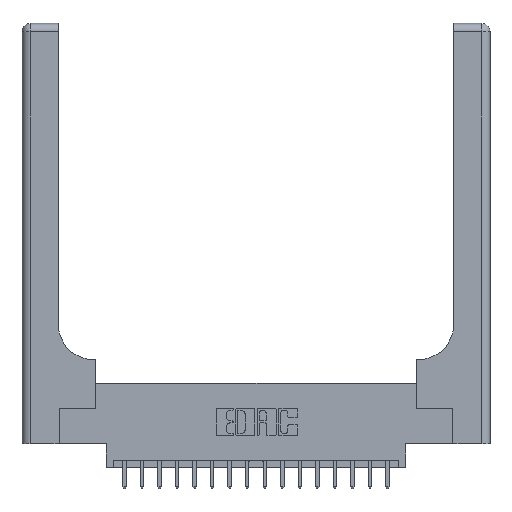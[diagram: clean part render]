
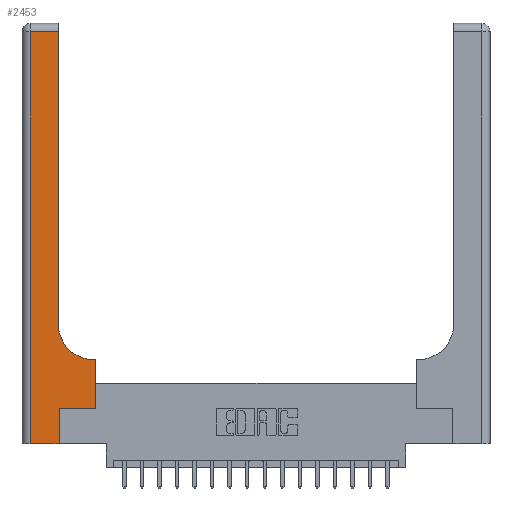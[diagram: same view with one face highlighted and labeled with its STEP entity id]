
A CAD part, top view. The second image highlights one B-rep face of the part: STEP entity #2453.
In plain terms, the highlighted planar face has unit normal (0, 0, 1).
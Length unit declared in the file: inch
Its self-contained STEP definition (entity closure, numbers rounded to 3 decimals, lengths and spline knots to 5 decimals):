
#224 = DIRECTION ( 'NONE',  ( 0., 1., 0. ) ) ;
#339 = CARTESIAN_POINT ( 'NONE',  ( 0.51, 0.85, 0.37 ) ) ;
#868 = VERTEX_POINT ( 'NONE', #2030 ) ;
#1755 = EDGE_CURVE ( 'NONE', #17602, #10268, #3141, .T. ) ;
#1922 = VECTOR ( 'NONE', #18468, 39.37008 ) ;
#1943 = CIRCLE ( 'NONE', #13120, 0.25 ) ;
#2030 = CARTESIAN_POINT ( 'NONE',  ( 0.528, 0.25, 0.37 ) ) ;
#2157 = CARTESIAN_POINT ( 'NONE',  ( 0.26, 2.94, 0.37 ) ) ;
#2203 = ORIENTED_EDGE ( 'NONE', *, *, #10490, .T. ) ;
#2453 = ADVANCED_FACE ( 'NONE', ( #17596 ), #16292, .F. ) ;
#2604 = CARTESIAN_POINT ( 'NONE',  ( 0., 3., 0.37 ) ) ;
#2752 = CARTESIAN_POINT ( 'NONE',  ( 0.265, 0.25, 0.37 ) ) ;
#2941 = VECTOR ( 'NONE', #11471, 39.37008 ) ;
#3141 = LINE ( 'NONE', #10660, #6651 ) ;
#3242 = ORIENTED_EDGE ( 'NONE', *, *, #4620, .T. ) ;
#4049 = CARTESIAN_POINT ( 'NONE',  ( 0., 0., 0.37 ) ) ;
#4089 = AXIS2_PLACEMENT_3D ( 'NONE', #2604, #8740, #15910 ) ;
#4101 = VERTEX_POINT ( 'NONE', #5188 ) ;
#4168 = VECTOR ( 'NONE', #9171, 39.37008 ) ;
#4620 = EDGE_CURVE ( 'NONE', #10268, #868, #8694, .T. ) ;
#4807 = VECTOR ( 'NONE', #8848, 39.37008 ) ;
#4898 = VERTEX_POINT ( 'NONE', #13884 ) ;
#5188 = CARTESIAN_POINT ( 'NONE',  ( 0.06, 2.94, 0.37 ) ) ;
#5408 = EDGE_LOOP ( 'NONE', ( #11699, #5452, #8083, #2203, #16127, #3242, #11478, #6878, #17930 ) ) ;
#5452 = ORIENTED_EDGE ( 'NONE', *, *, #7644, .T. ) ;
#5536 = CARTESIAN_POINT ( 'NONE',  ( 0.06, 3., 0.37 ) ) ;
#5556 = EDGE_CURVE ( 'NONE', #12656, #9653, #10816, .T. ) ;
#5921 = CARTESIAN_POINT ( 'NONE',  ( 0.06, 0., 0.37 ) ) ;
#6074 = VERTEX_POINT ( 'NONE', #2157 ) ;
#6420 = DIRECTION ( 'NONE',  ( 0., 0., -1. ) ) ;
#6651 = VECTOR ( 'NONE', #9278, 39.37008 ) ;
#6656 = EDGE_CURVE ( 'NONE', #4101, #14991, #19210, .T. ) ;
#6878 = ORIENTED_EDGE ( 'NONE', *, *, #5556, .T. ) ;
#7611 = LINE ( 'NONE', #18388, #17692 ) ;
#7644 = EDGE_CURVE ( 'NONE', #6074, #4101, #11165, .T. ) ;
#7708 = CARTESIAN_POINT ( 'NONE',  ( 0.26, 3., 0.37 ) ) ;
#8083 = ORIENTED_EDGE ( 'NONE', *, *, #6656, .T. ) ;
#8111 = CARTESIAN_POINT ( 'NONE',  ( 0.26, 0.6, 0.37 ) ) ;
#8381 = CARTESIAN_POINT ( 'NONE',  ( 0.528, 0.6, 0.37 ) ) ;
#8694 = LINE ( 'NONE', #19356, #11516 ) ;
#8740 = DIRECTION ( 'NONE',  ( 0., 0., -1. ) ) ;
#8848 = DIRECTION ( 'NONE',  ( 0., -1., 0. ) ) ;
#9171 = DIRECTION ( 'NONE',  ( -1., 0., 0. ) ) ;
#9278 = DIRECTION ( 'NONE',  ( 0., 1., 0. ) ) ;
#9653 = VERTEX_POINT ( 'NONE', #11040 ) ;
#10268 = VERTEX_POINT ( 'NONE', #2752 ) ;
#10490 = EDGE_CURVE ( 'NONE', #14991, #17602, #18935, .T. ) ;
#10660 = CARTESIAN_POINT ( 'NONE',  ( 0.265, 0., 0.37 ) ) ;
#10719 = LINE ( 'NONE', #7708, #15701 ) ;
#10723 = DIRECTION ( 'NONE',  ( 0., 1., 0. ) ) ;
#10816 = LINE ( 'NONE', #8111, #1922 ) ;
#11040 = CARTESIAN_POINT ( 'NONE',  ( 0.51, 0.6, 0.37 ) ) ;
#11165 = LINE ( 'NONE', #15438, #4168 ) ;
#11471 = DIRECTION ( 'NONE',  ( 1., 0., 0. ) ) ;
#11478 = ORIENTED_EDGE ( 'NONE', *, *, #12071, .T. ) ;
#11516 = VECTOR ( 'NONE', #16539, 39.37008 ) ;
#11699 = ORIENTED_EDGE ( 'NONE', *, *, #17885, .T. ) ;
#12071 = EDGE_CURVE ( 'NONE', #868, #12656, #7611, .T. ) ;
#12656 = VERTEX_POINT ( 'NONE', #8381 ) ;
#13120 = AXIS2_PLACEMENT_3D ( 'NONE', #339, #6420, #14313 ) ;
#13884 = CARTESIAN_POINT ( 'NONE',  ( 0.26, 0.85, 0.37 ) ) ;
#14313 = DIRECTION ( 'NONE',  ( 1., 0., 0. ) ) ;
#14991 = VERTEX_POINT ( 'NONE', #5921 ) ;
#15438 = CARTESIAN_POINT ( 'NONE',  ( 0., 2.94, 0.37 ) ) ;
#15701 = VECTOR ( 'NONE', #224, 39.37008 ) ;
#15910 = DIRECTION ( 'NONE',  ( -1., 0., 0. ) ) ;
#16127 = ORIENTED_EDGE ( 'NONE', *, *, #1755, .T. ) ;
#16184 = CARTESIAN_POINT ( 'NONE',  ( 0.265, 0., 0.37 ) ) ;
#16292 = PLANE ( 'NONE',  #4089 ) ;
#16300 = EDGE_CURVE ( 'NONE', #9653, #4898, #1943, .T. ) ;
#16539 = DIRECTION ( 'NONE',  ( 1., 0., 0. ) ) ;
#17596 = FACE_OUTER_BOUND ( 'NONE', #5408, .T. ) ;
#17602 = VERTEX_POINT ( 'NONE', #16184 ) ;
#17692 = VECTOR ( 'NONE', #10723, 39.37008 ) ;
#17885 = EDGE_CURVE ( 'NONE', #4898, #6074, #10719, .T. ) ;
#17930 = ORIENTED_EDGE ( 'NONE', *, *, #16300, .T. ) ;
#18388 = CARTESIAN_POINT ( 'NONE',  ( 0.528, 0.25, 0.37 ) ) ;
#18468 = DIRECTION ( 'NONE',  ( -1., 0., 0. ) ) ;
#18935 = LINE ( 'NONE', #4049, #2941 ) ;
#19210 = LINE ( 'NONE', #5536, #4807 ) ;
#19356 = CARTESIAN_POINT ( 'NONE',  ( 0.265, 0.25, 0.37 ) ) ;
